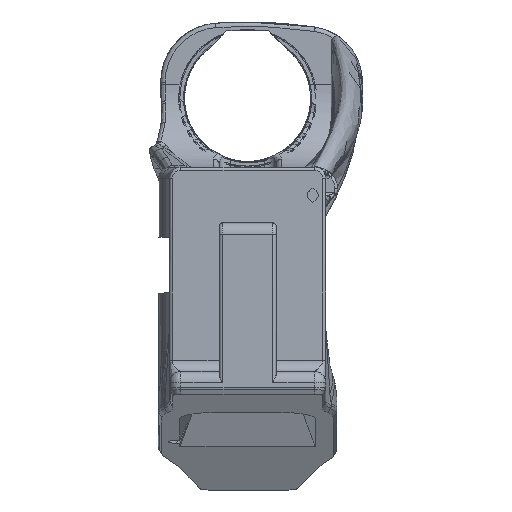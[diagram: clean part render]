
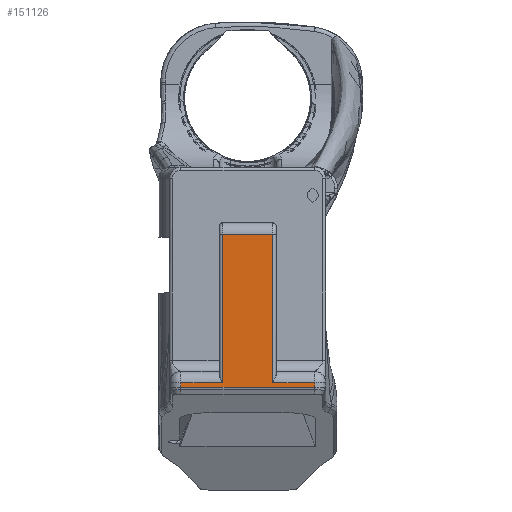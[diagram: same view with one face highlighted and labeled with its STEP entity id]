
A CAD part, top view. The second image highlights one B-rep face of the part: STEP entity #151126.
In plain terms, the highlighted planar face has unit normal (0, 0, 1).
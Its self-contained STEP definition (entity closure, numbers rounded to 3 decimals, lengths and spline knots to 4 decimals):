
#2703 = DIRECTION ( 'NONE',  ( 0., 1., 0. ) ) ;
#4283 = EDGE_CURVE ( 'NONE', #198380, #217261, #152723, .T. ) ;
#5479 = ORIENTED_EDGE ( 'NONE', *, *, #170017, .T. ) ;
#10558 = DIRECTION ( 'NONE',  ( 0., 1., 0. ) ) ;
#11734 = VECTOR ( 'NONE', #119556, 39.3701 ) ;
#15502 = ORIENTED_EDGE ( 'NONE', *, *, #137846, .T. ) ;
#18338 = DIRECTION ( 'NONE',  ( 1., 0., 0. ) ) ;
#18675 = LINE ( 'NONE', #73868, #91553 ) ;
#19236 = VECTOR ( 'NONE', #18338, 39.3701 ) ;
#24124 = LINE ( 'NONE', #108253, #100903 ) ;
#37117 = PLANE ( 'NONE',  #152939 ) ;
#54754 = EDGE_LOOP ( 'NONE', ( #180107, #15502, #5479, #171839, #62720, #176985, #153483, #98760 ) ) ;
#58198 = EDGE_CURVE ( 'NONE', #195838, #142647, #18675, .T. ) ;
#62720 = ORIENTED_EDGE ( 'NONE', *, *, #67938, .T. ) ;
#66788 = LINE ( 'NONE', #216423, #186696 ) ;
#67938 = EDGE_CURVE ( 'NONE', #142647, #198380, #24124, .T. ) ;
#72114 = DIRECTION ( 'NONE',  ( -1., 0., 0. ) ) ;
#72336 = LINE ( 'NONE', #147116, #19236 ) ;
#73868 = CARTESIAN_POINT ( 'NONE',  ( 0.255, -1.9323, 6.65 ) ) ;
#91553 = VECTOR ( 'NONE', #203894, 39.3701 ) ;
#93501 = FACE_OUTER_BOUND ( 'NONE', #54754, .T. ) ;
#98760 = ORIENTED_EDGE ( 'NONE', *, *, #175610, .T. ) ;
#100903 = VECTOR ( 'NONE', #10558, 39.3701 ) ;
#107673 = LINE ( 'NONE', #148094, #202474 ) ;
#108253 = CARTESIAN_POINT ( 'NONE',  ( 0.225, -2.0323, 6.65 ) ) ;
#119350 = CARTESIAN_POINT ( 'NONE',  ( -0.225, -0.6, 6.65 ) ) ;
#119556 = DIRECTION ( 'NONE',  ( -1., 0., 0. ) ) ;
#121267 = CARTESIAN_POINT ( 'NONE',  ( 0.6, -1.9323, 6.65 ) ) ;
#125110 = CARTESIAN_POINT ( 'NONE',  ( -0.6, -1.9765, 6.65 ) ) ;
#132410 = LINE ( 'NONE', #208466, #163050 ) ;
#137846 = EDGE_CURVE ( 'NONE', #208541, #161570, #72336, .T. ) ;
#138957 = VERTEX_POINT ( 'NONE', #161352 ) ;
#142647 = VERTEX_POINT ( 'NONE', #152517 ) ;
#147116 = CARTESIAN_POINT ( 'NONE',  ( 0.6, -1.9765, 6.65 ) ) ;
#148094 = CARTESIAN_POINT ( 'NONE',  ( 0.255, -1.9323, 6.65 ) ) ;
#149888 = CARTESIAN_POINT ( 'NONE',  ( 0.255, -2.0323, 6.65 ) ) ;
#151126 = ADVANCED_FACE ( 'NONE', ( #93501 ), #37117, .F. ) ;
#152517 = CARTESIAN_POINT ( 'NONE',  ( 0.225, -1.9323, 6.65 ) ) ;
#152698 = DIRECTION ( 'NONE',  ( 0., -1., 0. ) ) ;
#152723 = LINE ( 'NONE', #231215, #11734 ) ;
#152939 = AXIS2_PLACEMENT_3D ( 'NONE', #149888, #170699, #2703 ) ;
#153483 = ORIENTED_EDGE ( 'NONE', *, *, #177092, .T. ) ;
#154834 = CARTESIAN_POINT ( 'NONE',  ( -0.6, -1.9323, 6.65 ) ) ;
#161352 = CARTESIAN_POINT ( 'NONE',  ( -0.225, -1.9323, 6.65 ) ) ;
#161570 = VERTEX_POINT ( 'NONE', #220029 ) ;
#163050 = VECTOR ( 'NONE', #191293, 39.3701 ) ;
#166904 = VECTOR ( 'NONE', #152698, 39.3701 ) ;
#170017 = EDGE_CURVE ( 'NONE', #161570, #195838, #132410, .T. ) ;
#170699 = DIRECTION ( 'NONE',  ( 0., 0., -1. ) ) ;
#171096 = EDGE_CURVE ( 'NONE', #182399, #208541, #213997, .T. ) ;
#171839 = ORIENTED_EDGE ( 'NONE', *, *, #58198, .T. ) ;
#175610 = EDGE_CURVE ( 'NONE', #138957, #182399, #107673, .T. ) ;
#176985 = ORIENTED_EDGE ( 'NONE', *, *, #4283, .T. ) ;
#177092 = EDGE_CURVE ( 'NONE', #217261, #138957, #66788, .T. ) ;
#178918 = CARTESIAN_POINT ( 'NONE',  ( 0.225, -0.6, 6.65 ) ) ;
#179598 = DIRECTION ( 'NONE',  ( 0., -1., 0. ) ) ;
#180107 = ORIENTED_EDGE ( 'NONE', *, *, #171096, .T. ) ;
#182399 = VERTEX_POINT ( 'NONE', #154834 ) ;
#186696 = VECTOR ( 'NONE', #179598, 39.3701 ) ;
#189532 = CARTESIAN_POINT ( 'NONE',  ( -0.6, -2.0323, 6.65 ) ) ;
#191293 = DIRECTION ( 'NONE',  ( 0., 1., 0. ) ) ;
#195838 = VERTEX_POINT ( 'NONE', #121267 ) ;
#198380 = VERTEX_POINT ( 'NONE', #178918 ) ;
#202474 = VECTOR ( 'NONE', #72114, 39.3701 ) ;
#203894 = DIRECTION ( 'NONE',  ( -1., 0., 0. ) ) ;
#208466 = CARTESIAN_POINT ( 'NONE',  ( 0.6, -1.8323, 6.65 ) ) ;
#208541 = VERTEX_POINT ( 'NONE', #125110 ) ;
#213997 = LINE ( 'NONE', #189532, #166904 ) ;
#216423 = CARTESIAN_POINT ( 'NONE',  ( -0.225, -1.8323, 6.65 ) ) ;
#217261 = VERTEX_POINT ( 'NONE', #119350 ) ;
#220029 = CARTESIAN_POINT ( 'NONE',  ( 0.6, -1.9765, 6.65 ) ) ;
#231215 = CARTESIAN_POINT ( 'NONE',  ( 0.255, -0.6, 6.65 ) ) ;
